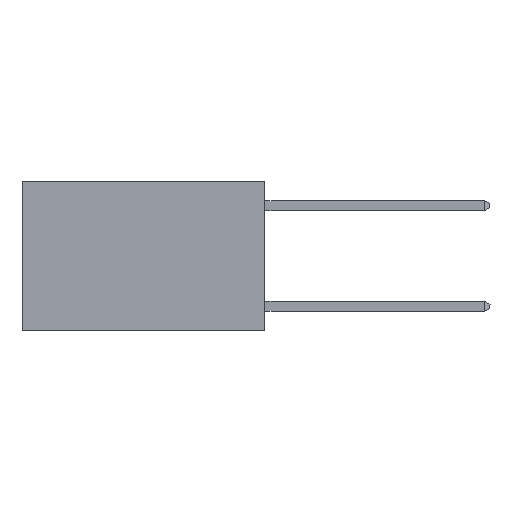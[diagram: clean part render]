
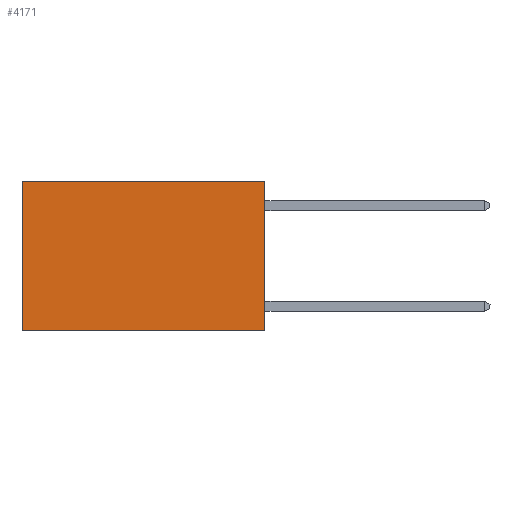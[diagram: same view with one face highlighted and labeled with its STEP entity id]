
A CAD part, left-side view. The second image highlights one B-rep face of the part: STEP entity #4171.
In plain terms, the highlighted planar face has unit normal (-1, 0, 0).
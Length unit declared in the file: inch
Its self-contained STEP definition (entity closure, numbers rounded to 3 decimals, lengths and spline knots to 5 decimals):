
#562 = CARTESIAN_POINT ( 'NONE',  ( 0.2625, 0.6, 0. ) ) ;
#687 = ORIENTED_EDGE ( 'NONE', *, *, #1491, .T. ) ;
#753 = ORIENTED_EDGE ( 'NONE', *, *, #4460, .F. ) ;
#967 = PLANE ( 'NONE',  #3025 ) ;
#1132 = ORIENTED_EDGE ( 'NONE', *, *, #1295, .F. ) ;
#1256 = ORIENTED_EDGE ( 'NONE', *, *, #4347, .T. ) ;
#1295 = EDGE_CURVE ( 'NONE', #6576, #1401, #5637, .T. ) ;
#1401 = VERTEX_POINT ( 'NONE', #6413 ) ;
#1491 = EDGE_CURVE ( 'NONE', #2443, #7358, #9104, .T. ) ;
#1499 = VECTOR ( 'NONE', #5966, 39.37008 ) ;
#1613 = VECTOR ( 'NONE', #3778, 39.37008 ) ;
#1744 = DIRECTION ( 'NONE',  ( 0., 0., -1. ) ) ;
#1851 = EDGE_LOOP ( 'NONE', ( #687, #753, #1132, #1256 ) ) ;
#1903 = CARTESIAN_POINT ( 'NONE',  ( 0.2625, 0., 0. ) ) ;
#1905 = VECTOR ( 'NONE', #4902, 39.37008 ) ;
#2443 = VERTEX_POINT ( 'NONE', #4614 ) ;
#3025 = AXIS2_PLACEMENT_3D ( 'NONE', #8882, #6020, #1744 ) ;
#3175 = CARTESIAN_POINT ( 'NONE',  ( 0.2625, 0., 0. ) ) ;
#3588 = LINE ( 'NONE', #9139, #1905 ) ;
#3778 = DIRECTION ( 'NONE',  ( 0., 0., -1. ) ) ;
#3940 = FACE_OUTER_BOUND ( 'NONE', #1851, .T. ) ;
#4171 = ADVANCED_FACE ( 'NONE', ( #3940 ), #967, .F. ) ;
#4347 = EDGE_CURVE ( 'NONE', #6576, #2443, #6386, .T. ) ;
#4460 = EDGE_CURVE ( 'NONE', #1401, #7358, #3588, .T. ) ;
#4614 = CARTESIAN_POINT ( 'NONE',  ( 0.2625, 0.6, 0. ) ) ;
#4724 = VECTOR ( 'NONE', #8349, 39.37008 ) ;
#4771 = CARTESIAN_POINT ( 'NONE',  ( 0.2625, 0.6, -0.37 ) ) ;
#4902 = DIRECTION ( 'NONE',  ( 0., 1., 0. ) ) ;
#5637 = LINE ( 'NONE', #9176, #1613 ) ;
#5966 = DIRECTION ( 'NONE',  ( 0., 0., -1. ) ) ;
#6020 = DIRECTION ( 'NONE',  ( 1., 0., 0. ) ) ;
#6386 = LINE ( 'NONE', #1903, #4724 ) ;
#6413 = CARTESIAN_POINT ( 'NONE',  ( 0.2625, 0., -0.37 ) ) ;
#6576 = VERTEX_POINT ( 'NONE', #3175 ) ;
#7358 = VERTEX_POINT ( 'NONE', #4771 ) ;
#8349 = DIRECTION ( 'NONE',  ( 0., 1., 0. ) ) ;
#8882 = CARTESIAN_POINT ( 'NONE',  ( 0.2625, 0., 0. ) ) ;
#9104 = LINE ( 'NONE', #562, #1499 ) ;
#9139 = CARTESIAN_POINT ( 'NONE',  ( 0.2625, 0., -0.37 ) ) ;
#9176 = CARTESIAN_POINT ( 'NONE',  ( 0.2625, 0., 0. ) ) ;
